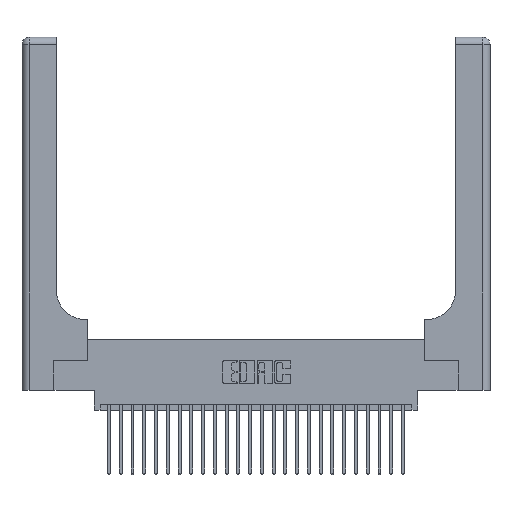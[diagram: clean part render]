
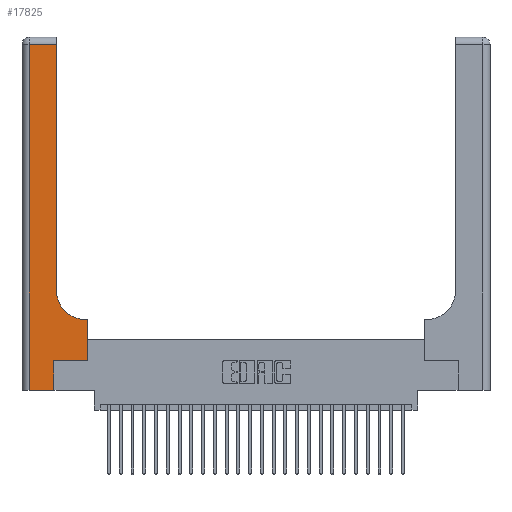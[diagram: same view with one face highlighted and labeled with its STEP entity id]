
A CAD part, top view. The second image highlights one B-rep face of the part: STEP entity #17825.
In plain terms, the highlighted planar face has unit normal (0, 0, 1).
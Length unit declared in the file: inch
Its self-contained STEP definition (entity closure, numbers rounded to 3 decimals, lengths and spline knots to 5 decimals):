
#386 = CARTESIAN_POINT ( 'NONE',  ( 0.2915, 3., 0.37 ) ) ;
#1999 = CARTESIAN_POINT ( 'NONE',  ( 0., 2.94, 0.37 ) ) ;
#2122 = CARTESIAN_POINT ( 'NONE',  ( 0.5585, 0.25, 0.37 ) ) ;
#2137 = CARTESIAN_POINT ( 'NONE',  ( 0.5415, 0.6, 0.37 ) ) ;
#2614 = CARTESIAN_POINT ( 'NONE',  ( 0.2915, 2.94, 0.37 ) ) ;
#3503 = CARTESIAN_POINT ( 'NONE',  ( 0.06, 3., 0.37 ) ) ;
#4186 = DIRECTION ( 'NONE',  ( -1., 0., 0. ) ) ;
#5034 = VERTEX_POINT ( 'NONE', #26529 ) ;
#5221 = EDGE_CURVE ( 'NONE', #5034, #5919, #20740, .T. ) ;
#5690 = CARTESIAN_POINT ( 'NONE',  ( 0., 0., 0.37 ) ) ;
#5748 = FACE_OUTER_BOUND ( 'NONE', #15469, .T. ) ;
#5919 = VERTEX_POINT ( 'NONE', #20556 ) ;
#6528 = EDGE_CURVE ( 'NONE', #25890, #23776, #7202, .T. ) ;
#6554 = VECTOR ( 'NONE', #9842, 39.37008 ) ;
#7202 = LINE ( 'NONE', #20720, #23711 ) ;
#7834 = EDGE_CURVE ( 'NONE', #5919, #25890, #16897, .T. ) ;
#7893 = AXIS2_PLACEMENT_3D ( 'NONE', #8237, #23317, #10388 ) ;
#7974 = AXIS2_PLACEMENT_3D ( 'NONE', #18348, #21007, #8071 ) ;
#8071 = DIRECTION ( 'NONE',  ( -1., 0., 0. ) ) ;
#8115 = VERTEX_POINT ( 'NONE', #21850 ) ;
#8237 = CARTESIAN_POINT ( 'NONE',  ( 0.5415, 0.85, 0.37 ) ) ;
#8927 = VERTEX_POINT ( 'NONE', #2614 ) ;
#9572 = ORIENTED_EDGE ( 'NONE', *, *, #12429, .T. ) ;
#9810 = VECTOR ( 'NONE', #10045, 39.37008 ) ;
#9842 = DIRECTION ( 'NONE',  ( 0., -1., 0. ) ) ;
#10045 = DIRECTION ( 'NONE',  ( 0., 1., 0. ) ) ;
#10388 = DIRECTION ( 'NONE',  ( 1., 0., 0. ) ) ;
#10528 = EDGE_CURVE ( 'NONE', #16034, #22454, #25758, .T. ) ;
#10867 = VERTEX_POINT ( 'NONE', #24888 ) ;
#11576 = ORIENTED_EDGE ( 'NONE', *, *, #18511, .T. ) ;
#11604 = ORIENTED_EDGE ( 'NONE', *, *, #17037, .T. ) ;
#12429 = EDGE_CURVE ( 'NONE', #22454, #10867, #25644, .T. ) ;
#12775 = VECTOR ( 'NONE', #13226, 39.37008 ) ;
#13226 = DIRECTION ( 'NONE',  ( 0., 1., 0. ) ) ;
#13732 = EDGE_CURVE ( 'NONE', #8927, #8115, #21175, .T. ) ;
#14326 = ORIENTED_EDGE ( 'NONE', *, *, #7834, .T. ) ;
#15469 = EDGE_LOOP ( 'NONE', ( #11604, #21785, #24113, #25820, #14326, #23097, #11576, #21751, #9572 ) ) ;
#16034 = VERTEX_POINT ( 'NONE', #27454 ) ;
#16097 = VECTOR ( 'NONE', #17018, 39.37008 ) ;
#16897 = LINE ( 'NONE', #25157, #9810 ) ;
#17018 = DIRECTION ( 'NONE',  ( -1., 0., 0. ) ) ;
#17037 = EDGE_CURVE ( 'NONE', #10867, #8927, #18559, .T. ) ;
#17825 = ADVANCED_FACE ( 'NONE', ( #5748 ), #18818, .F. ) ;
#18027 = LINE ( 'NONE', #3503, #6554 ) ;
#18348 = CARTESIAN_POINT ( 'NONE',  ( 0., 3., 0.37 ) ) ;
#18511 = EDGE_CURVE ( 'NONE', #23776, #16034, #24572, .T. ) ;
#18559 = LINE ( 'NONE', #386, #12775 ) ;
#18818 = PLANE ( 'NONE',  #7974 ) ;
#19246 = CARTESIAN_POINT ( 'NONE',  ( 0.2915, 0.6, 0.37 ) ) ;
#20444 = CARTESIAN_POINT ( 'NONE',  ( 0.269, 0.25, 0.37 ) ) ;
#20556 = CARTESIAN_POINT ( 'NONE',  ( 0.269, 0., 0.37 ) ) ;
#20720 = CARTESIAN_POINT ( 'NONE',  ( 0.269, 0.25, 0.37 ) ) ;
#20740 = LINE ( 'NONE', #5690, #26479 ) ;
#20770 = DIRECTION ( 'NONE',  ( 1., 0., 0. ) ) ;
#20974 = DIRECTION ( 'NONE',  ( 0., 1., 0. ) ) ;
#21007 = DIRECTION ( 'NONE',  ( 0., 0., -1. ) ) ;
#21175 = LINE ( 'NONE', #1999, #16097 ) ;
#21363 = VECTOR ( 'NONE', #4186, 39.37008 ) ;
#21751 = ORIENTED_EDGE ( 'NONE', *, *, #10528, .T. ) ;
#21785 = ORIENTED_EDGE ( 'NONE', *, *, #13732, .T. ) ;
#21850 = CARTESIAN_POINT ( 'NONE',  ( 0.06, 2.94, 0.37 ) ) ;
#22454 = VERTEX_POINT ( 'NONE', #2137 ) ;
#23097 = ORIENTED_EDGE ( 'NONE', *, *, #6528, .T. ) ;
#23317 = DIRECTION ( 'NONE',  ( 0., 0., -1. ) ) ;
#23711 = VECTOR ( 'NONE', #27117, 39.37008 ) ;
#23776 = VERTEX_POINT ( 'NONE', #2122 ) ;
#23896 = VECTOR ( 'NONE', #20974, 39.37008 ) ;
#24113 = ORIENTED_EDGE ( 'NONE', *, *, #27839, .T. ) ;
#24572 = LINE ( 'NONE', #27379, #23896 ) ;
#24888 = CARTESIAN_POINT ( 'NONE',  ( 0.2915, 0.85, 0.37 ) ) ;
#25157 = CARTESIAN_POINT ( 'NONE',  ( 0.269, 0., 0.37 ) ) ;
#25644 = CIRCLE ( 'NONE', #7893, 0.25 ) ;
#25758 = LINE ( 'NONE', #19246, #21363 ) ;
#25820 = ORIENTED_EDGE ( 'NONE', *, *, #5221, .T. ) ;
#25890 = VERTEX_POINT ( 'NONE', #20444 ) ;
#26479 = VECTOR ( 'NONE', #20770, 39.37008 ) ;
#26529 = CARTESIAN_POINT ( 'NONE',  ( 0.06, 0., 0.37 ) ) ;
#27117 = DIRECTION ( 'NONE',  ( 1., 0., 0. ) ) ;
#27379 = CARTESIAN_POINT ( 'NONE',  ( 0.5585, 0.25, 0.37 ) ) ;
#27454 = CARTESIAN_POINT ( 'NONE',  ( 0.5585, 0.6, 0.37 ) ) ;
#27839 = EDGE_CURVE ( 'NONE', #8115, #5034, #18027, .T. ) ;
